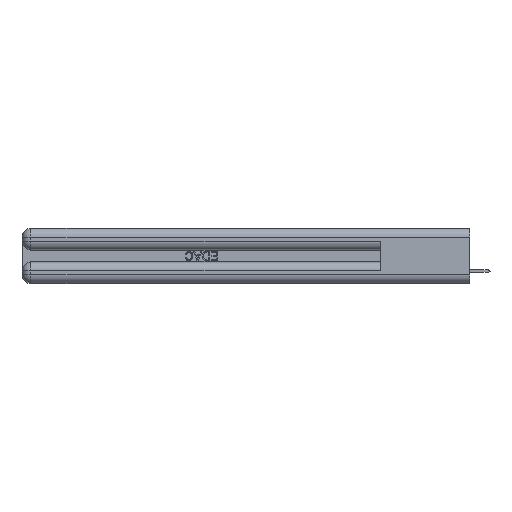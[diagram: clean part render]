
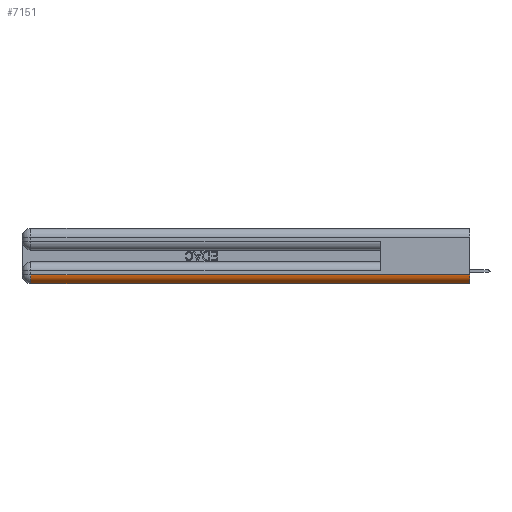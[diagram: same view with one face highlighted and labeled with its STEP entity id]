
A CAD part, left-side view. The second image highlights one B-rep face of the part: STEP entity #7151.
In plain terms, the highlighted cylindrical face has radius 1.524 mm (diameter 3.048 mm), a partial arc.
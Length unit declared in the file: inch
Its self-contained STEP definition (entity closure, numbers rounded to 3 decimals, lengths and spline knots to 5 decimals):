
#657 = VERTEX_POINT ( 'NONE', #33382 ) ;
#1147 = VERTEX_POINT ( 'NONE', #25199 ) ;
#3641 = AXIS2_PLACEMENT_3D ( 'NONE', #11345, #20921, #34864 ) ;
#5339 = EDGE_CURVE ( 'NONE', #657, #33967, #22405, .T. ) ;
#5738 = CYLINDRICAL_SURFACE ( 'NONE', #14213, 0.06 ) ;
#6497 = CARTESIAN_POINT ( 'NONE',  ( 0., 0., 0.06 ) ) ;
#6714 = ORIENTED_EDGE ( 'NONE', *, *, #19799, .F. ) ;
#7151 = ADVANCED_FACE ( 'NONE', ( #35583 ), #5738, .T. ) ;
#9226 = DIRECTION ( 'NONE',  ( 0., 1., 0. ) ) ;
#9907 = CARTESIAN_POINT ( 'NONE',  ( 0.06, 3., 0. ) ) ;
#11345 = CARTESIAN_POINT ( 'NONE',  ( 0.06, 2.94, 0.06 ) ) ;
#13268 = VECTOR ( 'NONE', #23184, 39.37008 ) ;
#14213 = AXIS2_PLACEMENT_3D ( 'NONE', #39063, #9226, #36015 ) ;
#15590 = LINE ( 'NONE', #9907, #13268 ) ;
#19799 = EDGE_CURVE ( 'NONE', #24183, #1147, #30586, .T. ) ;
#20921 = DIRECTION ( 'NONE',  ( 0., 1., 0. ) ) ;
#20954 = EDGE_CURVE ( 'NONE', #1147, #657, #15590, .T. ) ;
#22405 = CIRCLE ( 'NONE', #3641, 0.06 ) ;
#23184 = DIRECTION ( 'NONE',  ( 0., 1., 0. ) ) ;
#23377 = ORIENTED_EDGE ( 'NONE', *, *, #29658, .F. ) ;
#23614 = DIRECTION ( 'NONE',  ( 0., -1., 0. ) ) ;
#23821 = EDGE_LOOP ( 'NONE', ( #6714, #23377, #34937, #36465 ) ) ;
#23973 = DIRECTION ( 'NONE',  ( 0., -1., 0. ) ) ;
#24048 = DIRECTION ( 'NONE',  ( 0., 0., 1. ) ) ;
#24183 = VERTEX_POINT ( 'NONE', #6497 ) ;
#24350 = CARTESIAN_POINT ( 'NONE',  ( 0., 2.94, 0.06 ) ) ;
#25199 = CARTESIAN_POINT ( 'NONE',  ( 0.06, 0., 0. ) ) ;
#29658 = EDGE_CURVE ( 'NONE', #33967, #24183, #30068, .T. ) ;
#29861 = CARTESIAN_POINT ( 'NONE',  ( 0., 0., 0.06 ) ) ;
#30068 = LINE ( 'NONE', #29861, #42302 ) ;
#30586 = CIRCLE ( 'NONE', #35451, 0.06 ) ;
#33382 = CARTESIAN_POINT ( 'NONE',  ( 0.06, 2.94, 0. ) ) ;
#33967 = VERTEX_POINT ( 'NONE', #24350 ) ;
#34864 = DIRECTION ( 'NONE',  ( 0., 0., 1. ) ) ;
#34937 = ORIENTED_EDGE ( 'NONE', *, *, #5339, .F. ) ;
#35451 = AXIS2_PLACEMENT_3D ( 'NONE', #39735, #23614, #24048 ) ;
#35583 = FACE_OUTER_BOUND ( 'NONE', #23821, .T. ) ;
#36015 = DIRECTION ( 'NONE',  ( 0., 0., 1. ) ) ;
#36465 = ORIENTED_EDGE ( 'NONE', *, *, #20954, .F. ) ;
#39063 = CARTESIAN_POINT ( 'NONE',  ( 0.06, 0., 0.06 ) ) ;
#39735 = CARTESIAN_POINT ( 'NONE',  ( 0.06, 0., 0.06 ) ) ;
#42302 = VECTOR ( 'NONE', #23973, 39.37008 ) ;
